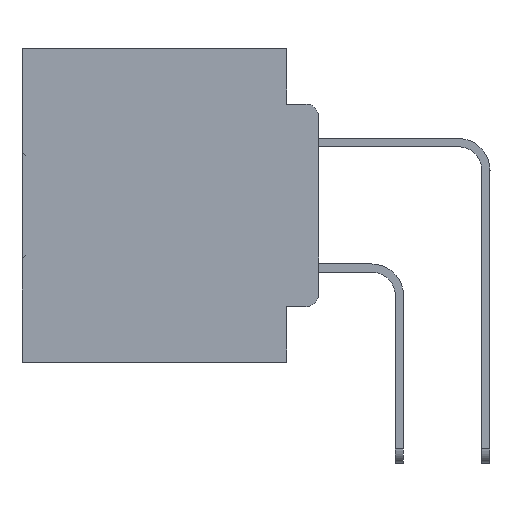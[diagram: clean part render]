
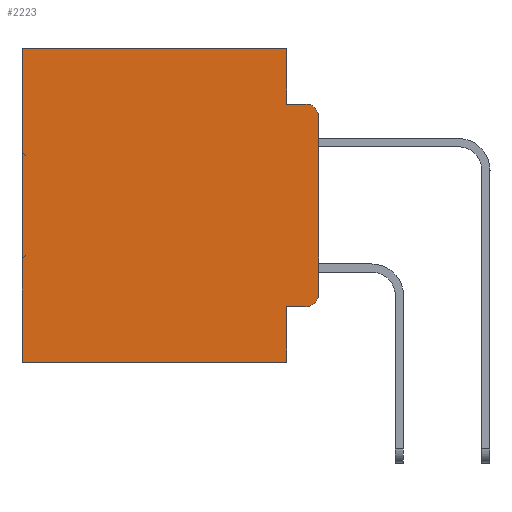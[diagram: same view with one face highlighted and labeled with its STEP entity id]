
A CAD part, left-side view. The second image highlights one B-rep face of the part: STEP entity #2223.
In plain terms, the highlighted planar face has unit normal (-1, 0, 0).
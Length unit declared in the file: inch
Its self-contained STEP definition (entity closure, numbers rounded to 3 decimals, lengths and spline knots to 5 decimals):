
#519 = EDGE_CURVE ( 'NONE', #24739, #12899, #23767, .T. ) ;
#1876 = CIRCLE ( 'NONE', #21946, 0.02 ) ;
#1954 = CARTESIAN_POINT ( 'NONE',  ( 0.298, 0.02, -0.4115 ) ) ;
#2140 = EDGE_CURVE ( 'NONE', #12899, #32760, #3791, .T. ) ;
#2223 = ADVANCED_FACE ( 'NONE', ( #14569 ), #22275, .F. ) ;
#3250 = DIRECTION ( 'NONE',  ( 1., 0., 0. ) ) ;
#3554 = AXIS2_PLACEMENT_3D ( 'NONE', #24013, #18812, #10718 ) ;
#3791 = LINE ( 'NONE', #33411, #18380 ) ;
#3946 = DIRECTION ( 'NONE',  ( 0., 0., -1. ) ) ;
#4226 = EDGE_CURVE ( 'NONE', #26684, #32760, #33357, .T. ) ;
#4635 = LINE ( 'NONE', #34094, #27641 ) ;
#4725 = ORIENTED_EDGE ( 'NONE', *, *, #4226, .T. ) ;
#4953 = EDGE_CURVE ( 'NONE', #24958, #7645, #1876, .T. ) ;
#5035 = VECTOR ( 'NONE', #32179, 39.37008 ) ;
#5092 = VERTEX_POINT ( 'NONE', #5213 ) ;
#5213 = CARTESIAN_POINT ( 'NONE',  ( 0.298, 0.051, -0.4115 ) ) ;
#5401 = EDGE_CURVE ( 'NONE', #5092, #24958, #4635, .T. ) ;
#6052 = CARTESIAN_POINT ( 'NONE',  ( 0.298, 0., 0. ) ) ;
#6319 = CARTESIAN_POINT ( 'NONE',  ( 0.298, 0., -0.3915 ) ) ;
#6827 = DIRECTION ( 'NONE',  ( 0., 0., -1. ) ) ;
#7645 = VERTEX_POINT ( 'NONE', #6319 ) ;
#8409 = ORIENTED_EDGE ( 'NONE', *, *, #34220, .F. ) ;
#9157 = LINE ( 'NONE', #34106, #28427 ) ;
#9671 = DIRECTION ( 'NONE',  ( 0., -1., 0. ) ) ;
#10493 = ORIENTED_EDGE ( 'NONE', *, *, #2140, .F. ) ;
#10502 = VECTOR ( 'NONE', #25094, 39.37008 ) ;
#10718 = DIRECTION ( 'NONE',  ( 0., 0., -1. ) ) ;
#11594 = VERTEX_POINT ( 'NONE', #19927 ) ;
#11950 = EDGE_CURVE ( 'NONE', #24739, #31863, #21855, .T. ) ;
#12231 = CARTESIAN_POINT ( 'NONE',  ( 0.298, 0.473, 0. ) ) ;
#12899 = VERTEX_POINT ( 'NONE', #22622 ) ;
#14387 = CARTESIAN_POINT ( 'NONE',  ( 0.298, 0., 0. ) ) ;
#14569 = FACE_OUTER_BOUND ( 'NONE', #24542, .T. ) ;
#16039 = EDGE_CURVE ( 'NONE', #26684, #7645, #17451, .T. ) ;
#17178 = ORIENTED_EDGE ( 'NONE', *, *, #4953, .T. ) ;
#17446 = CARTESIAN_POINT ( 'NONE',  ( 0.298, 0., 0. ) ) ;
#17451 = LINE ( 'NONE', #14387, #30801 ) ;
#17840 = LINE ( 'NONE', #18182, #5035 ) ;
#17966 = ORIENTED_EDGE ( 'NONE', *, *, #5401, .T. ) ;
#18182 = CARTESIAN_POINT ( 'NONE',  ( 0.298, 0.473, 0. ) ) ;
#18380 = VECTOR ( 'NONE', #28210, 39.37008 ) ;
#18812 = DIRECTION ( 'NONE',  ( -1., 0., 0. ) ) ;
#19410 = CARTESIAN_POINT ( 'NONE',  ( 0.298, 0.051, -0.5 ) ) ;
#19692 = ORIENTED_EDGE ( 'NONE', *, *, #27790, .F. ) ;
#19927 = CARTESIAN_POINT ( 'NONE',  ( 0.298, 0.473, -0.5 ) ) ;
#20611 = VECTOR ( 'NONE', #21241, 39.37008 ) ;
#21241 = DIRECTION ( 'NONE',  ( 0., 1., 0. ) ) ;
#21855 = LINE ( 'NONE', #6052, #10502 ) ;
#21946 = AXIS2_PLACEMENT_3D ( 'NONE', #28744, #23363, #26225 ) ;
#21950 = DIRECTION ( 'NONE',  ( 0., 0., -1. ) ) ;
#22132 = CARTESIAN_POINT ( 'NONE',  ( 0.298, 0.051, 0. ) ) ;
#22275 = PLANE ( 'NONE',  #24484 ) ;
#22622 = CARTESIAN_POINT ( 'NONE',  ( 0.298, 0.051, -0.0885 ) ) ;
#23351 = ORIENTED_EDGE ( 'NONE', *, *, #11950, .T. ) ;
#23363 = DIRECTION ( 'NONE',  ( -1., 0., 0. ) ) ;
#23767 = LINE ( 'NONE', #34707, #25990 ) ;
#24013 = CARTESIAN_POINT ( 'NONE',  ( 0.298, 0.02, -0.1085 ) ) ;
#24484 = AXIS2_PLACEMENT_3D ( 'NONE', #17446, #3250, #25157 ) ;
#24542 = EDGE_LOOP ( 'NONE', ( #25100, #4725, #10493, #34243, #23351, #26336, #8409, #19692, #17966, #17178 ) ) ;
#24739 = VERTEX_POINT ( 'NONE', #22132 ) ;
#24958 = VERTEX_POINT ( 'NONE', #1954 ) ;
#25094 = DIRECTION ( 'NONE',  ( 0., 1., 0. ) ) ;
#25100 = ORIENTED_EDGE ( 'NONE', *, *, #16039, .F. ) ;
#25157 = DIRECTION ( 'NONE',  ( 0., 0., -1. ) ) ;
#25990 = VECTOR ( 'NONE', #21950, 39.37008 ) ;
#26225 = DIRECTION ( 'NONE',  ( 0., 0., -1. ) ) ;
#26336 = ORIENTED_EDGE ( 'NONE', *, *, #30757, .T. ) ;
#26658 = VERTEX_POINT ( 'NONE', #19410 ) ;
#26684 = VERTEX_POINT ( 'NONE', #33937 ) ;
#27641 = VECTOR ( 'NONE', #9671, 39.37008 ) ;
#27790 = EDGE_CURVE ( 'NONE', #5092, #26658, #9157, .T. ) ;
#28210 = DIRECTION ( 'NONE',  ( 0., -1., 0. ) ) ;
#28427 = VECTOR ( 'NONE', #3946, 39.37008 ) ;
#28744 = CARTESIAN_POINT ( 'NONE',  ( 0.298, 0.02, -0.3915 ) ) ;
#29706 = CARTESIAN_POINT ( 'NONE',  ( 0.298, 0., -0.5 ) ) ;
#30757 = EDGE_CURVE ( 'NONE', #31863, #11594, #17840, .T. ) ;
#30801 = VECTOR ( 'NONE', #6827, 39.37008 ) ;
#31681 = CARTESIAN_POINT ( 'NONE',  ( 0.298, 0.02, -0.0885 ) ) ;
#31863 = VERTEX_POINT ( 'NONE', #12231 ) ;
#32179 = DIRECTION ( 'NONE',  ( 0., 0., -1. ) ) ;
#32760 = VERTEX_POINT ( 'NONE', #31681 ) ;
#33357 = CIRCLE ( 'NONE', #3554, 0.02 ) ;
#33411 = CARTESIAN_POINT ( 'NONE',  ( 0.298, 0.051, -0.0885 ) ) ;
#33937 = CARTESIAN_POINT ( 'NONE',  ( 0.298, 0., -0.1085 ) ) ;
#34094 = CARTESIAN_POINT ( 'NONE',  ( 0.298, 0.051, -0.4115 ) ) ;
#34106 = CARTESIAN_POINT ( 'NONE',  ( 0.298, 0.051, 0. ) ) ;
#34220 = EDGE_CURVE ( 'NONE', #26658, #11594, #35245, .T. ) ;
#34243 = ORIENTED_EDGE ( 'NONE', *, *, #519, .F. ) ;
#34707 = CARTESIAN_POINT ( 'NONE',  ( 0.298, 0.051, 0. ) ) ;
#35245 = LINE ( 'NONE', #29706, #20611 ) ;
